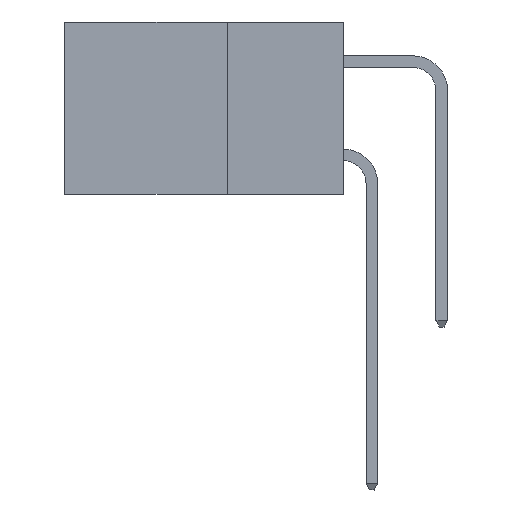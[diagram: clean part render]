
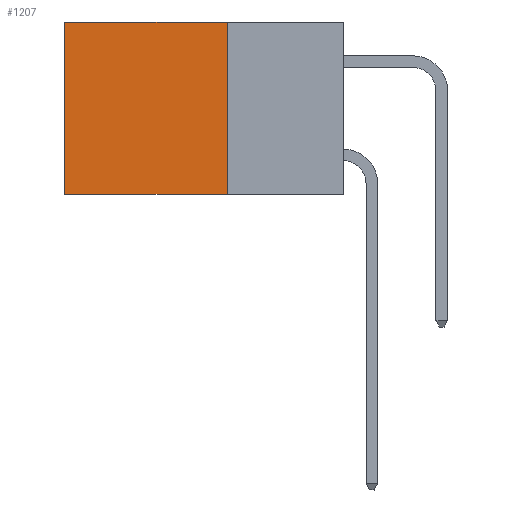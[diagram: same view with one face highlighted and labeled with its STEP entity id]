
A CAD part, left-side view. The second image highlights one B-rep face of the part: STEP entity #1207.
In plain terms, the highlighted planar face has unit normal (-1, 0, 0).
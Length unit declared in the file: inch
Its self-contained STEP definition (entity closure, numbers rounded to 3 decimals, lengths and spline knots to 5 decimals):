
#182 = DIRECTION ( 'NONE',  ( 0., 0., -1. ) ) ;
#1207 = ADVANCED_FACE ( 'NONE', ( #16252 ), #19861, .F. ) ;
#1628 = CARTESIAN_POINT ( 'NONE',  ( 0.2615, 0.6, -0.37 ) ) ;
#2623 = CARTESIAN_POINT ( 'NONE',  ( 0.2615, 0.25, -0.37 ) ) ;
#3362 = VERTEX_POINT ( 'NONE', #11481 ) ;
#3995 = DIRECTION ( 'NONE',  ( 0., 0., -1. ) ) ;
#4212 = EDGE_CURVE ( 'NONE', #10596, #3362, #4240, .T. ) ;
#4240 = LINE ( 'NONE', #4484, #13918 ) ;
#4484 = CARTESIAN_POINT ( 'NONE',  ( 0.2615, 0.25, -0.37 ) ) ;
#4735 = VERTEX_POINT ( 'NONE', #10169 ) ;
#6487 = EDGE_CURVE ( 'NONE', #4735, #22804, #9511, .T. ) ;
#6616 = ORIENTED_EDGE ( 'NONE', *, *, #23618, .T. ) ;
#7701 = CARTESIAN_POINT ( 'NONE',  ( 0.2615, 0.25, 0. ) ) ;
#8980 = DIRECTION ( 'NONE',  ( 1., 0., 0. ) ) ;
#9511 = LINE ( 'NONE', #1628, #9925 ) ;
#9651 = DIRECTION ( 'NONE',  ( 0., 1., 0. ) ) ;
#9925 = VECTOR ( 'NONE', #182, 39.37008 ) ;
#9952 = CARTESIAN_POINT ( 'NONE',  ( 0.2615, 0.6, -0.37 ) ) ;
#10169 = CARTESIAN_POINT ( 'NONE',  ( 0.2615, 0.6, 0. ) ) ;
#10486 = VECTOR ( 'NONE', #9651, 39.37008 ) ;
#10596 = VERTEX_POINT ( 'NONE', #17069 ) ;
#11481 = CARTESIAN_POINT ( 'NONE',  ( 0.2615, 0.25, -0.37 ) ) ;
#11840 = LINE ( 'NONE', #2623, #15166 ) ;
#12893 = EDGE_LOOP ( 'NONE', ( #22091, #23441, #16340, #6616 ) ) ;
#13918 = VECTOR ( 'NONE', #3995, 39.37008 ) ;
#14438 = DIRECTION ( 'NONE',  ( 0., 0., -1. ) ) ;
#15166 = VECTOR ( 'NONE', #19325, 39.37008 ) ;
#16252 = FACE_OUTER_BOUND ( 'NONE', #12893, .T. ) ;
#16264 = AXIS2_PLACEMENT_3D ( 'NONE', #18419, #8980, #14438 ) ;
#16340 = ORIENTED_EDGE ( 'NONE', *, *, #4212, .F. ) ;
#17069 = CARTESIAN_POINT ( 'NONE',  ( 0.2615, 0.25, 0. ) ) ;
#18419 = CARTESIAN_POINT ( 'NONE',  ( 0.2615, 0.25, -0.37 ) ) ;
#19325 = DIRECTION ( 'NONE',  ( 0., 1., 0. ) ) ;
#19861 = PLANE ( 'NONE',  #16264 ) ;
#20163 = LINE ( 'NONE', #7701, #10486 ) ;
#22091 = ORIENTED_EDGE ( 'NONE', *, *, #6487, .T. ) ;
#22804 = VERTEX_POINT ( 'NONE', #9952 ) ;
#23377 = EDGE_CURVE ( 'NONE', #3362, #22804, #11840, .T. ) ;
#23441 = ORIENTED_EDGE ( 'NONE', *, *, #23377, .F. ) ;
#23618 = EDGE_CURVE ( 'NONE', #10596, #4735, #20163, .T. ) ;
